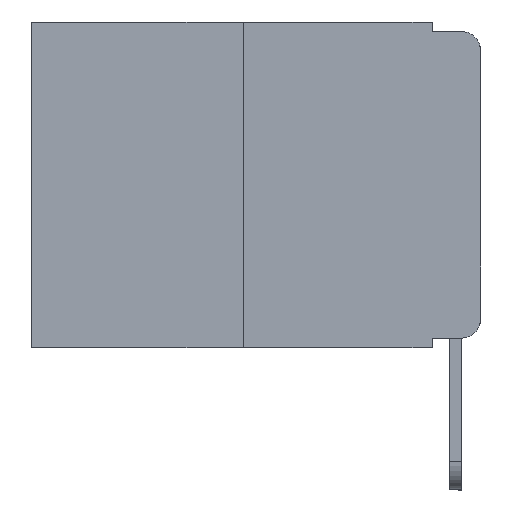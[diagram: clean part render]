
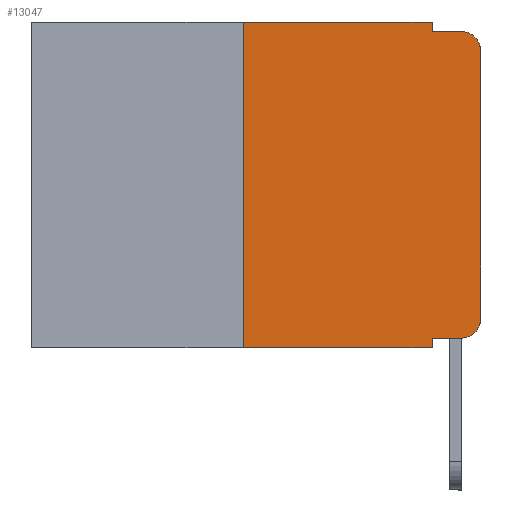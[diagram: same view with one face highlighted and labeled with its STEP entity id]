
A CAD part, left-side view. The second image highlights one B-rep face of the part: STEP entity #13047.
In plain terms, the highlighted planar face has unit normal (-1, 0, 0).
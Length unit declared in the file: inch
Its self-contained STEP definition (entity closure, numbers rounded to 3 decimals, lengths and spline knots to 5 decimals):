
#60 = CARTESIAN_POINT ( 'NONE',  ( 0., 0.02, -0.01 ) ) ;
#327 = FACE_OUTER_BOUND ( 'NONE', #13938, .T. ) ;
#675 = CARTESIAN_POINT ( 'NONE',  ( 0., 0., -0.313 ) ) ;
#951 = EDGE_CURVE ( 'NONE', #6253, #8660, #1093, .T. ) ;
#1003 = CARTESIAN_POINT ( 'NONE',  ( 0., 0., 0. ) ) ;
#1093 = LINE ( 'NONE', #10043, #1370 ) ;
#1110 = CARTESIAN_POINT ( 'NONE',  ( 0., 0.051, -0.333 ) ) ;
#1283 = DIRECTION ( 'NONE',  ( 0., 0., -1. ) ) ;
#1335 = CARTESIAN_POINT ( 'NONE',  ( 0., 0.051, -0.01 ) ) ;
#1370 = VECTOR ( 'NONE', #1283, 39.37008 ) ;
#1663 = ORIENTED_EDGE ( 'NONE', *, *, #7862, .T. ) ;
#1770 = VERTEX_POINT ( 'NONE', #11690 ) ;
#1880 = CIRCLE ( 'NONE', #13882, 0.02 ) ;
#1901 = VECTOR ( 'NONE', #13381, 39.37008 ) ;
#1945 = DIRECTION ( 'NONE',  ( 0., 0., -1. ) ) ;
#2068 = DIRECTION ( 'NONE',  ( -1., 0., 0. ) ) ;
#2071 = CARTESIAN_POINT ( 'NONE',  ( 0., 0.473, 0. ) ) ;
#2600 = EDGE_CURVE ( 'NONE', #15318, #6253, #12463, .T. ) ;
#2618 = DIRECTION ( 'NONE',  ( 0., 0., 1. ) ) ;
#3320 = DIRECTION ( 'NONE',  ( 0., 0., -1. ) ) ;
#3401 = LINE ( 'NONE', #13617, #16373 ) ;
#3673 = DIRECTION ( 'NONE',  ( 1., 0., 0. ) ) ;
#3693 = DIRECTION ( 'NONE',  ( 0., -1., 0. ) ) ;
#3809 = VECTOR ( 'NONE', #3693, 39.37008 ) ;
#4186 = AXIS2_PLACEMENT_3D ( 'NONE', #15248, #3673, #3320 ) ;
#4267 = CARTESIAN_POINT ( 'NONE',  ( 0., 0.02, -0.333 ) ) ;
#4283 = VECTOR ( 'NONE', #12015, 39.37008 ) ;
#4466 = EDGE_CURVE ( 'NONE', #13913, #15318, #17165, .T. ) ;
#4729 = CIRCLE ( 'NONE', #17966, 0.02 ) ;
#4837 = VERTEX_POINT ( 'NONE', #675 ) ;
#4962 = ORIENTED_EDGE ( 'NONE', *, *, #4466, .F. ) ;
#5260 = DIRECTION ( 'NONE',  ( 0., 0., -1. ) ) ;
#6099 = ORIENTED_EDGE ( 'NONE', *, *, #7632, .T. ) ;
#6197 = VERTEX_POINT ( 'NONE', #18984 ) ;
#6253 = VERTEX_POINT ( 'NONE', #16194 ) ;
#6338 = CARTESIAN_POINT ( 'NONE',  ( 0., 0.051, -0.333 ) ) ;
#6472 = EDGE_CURVE ( 'NONE', #10472, #4837, #4729, .T. ) ;
#6666 = ORIENTED_EDGE ( 'NONE', *, *, #14820, .F. ) ;
#6845 = CARTESIAN_POINT ( 'NONE',  ( 0., 0.25, 0. ) ) ;
#6918 = EDGE_CURVE ( 'NONE', #4837, #6197, #14202, .T. ) ;
#6941 = VECTOR ( 'NONE', #2618, 39.37008 ) ;
#7389 = CARTESIAN_POINT ( 'NONE',  ( 0., 0.25, 0. ) ) ;
#7553 = ORIENTED_EDGE ( 'NONE', *, *, #14374, .T. ) ;
#7632 = EDGE_CURVE ( 'NONE', #17494, #10472, #7686, .T. ) ;
#7686 = LINE ( 'NONE', #6338, #10735 ) ;
#7763 = ORIENTED_EDGE ( 'NONE', *, *, #951, .F. ) ;
#7862 = EDGE_CURVE ( 'NONE', #13913, #1770, #11926, .T. ) ;
#7932 = DIRECTION ( 'NONE',  ( 0., 0., -1. ) ) ;
#8291 = CARTESIAN_POINT ( 'NONE',  ( 0., 0.051, -0.01 ) ) ;
#8660 = VERTEX_POINT ( 'NONE', #8291 ) ;
#8730 = CARTESIAN_POINT ( 'NONE',  ( 0., 0.473, -0.343 ) ) ;
#9581 = VERTEX_POINT ( 'NONE', #60 ) ;
#9664 = DIRECTION ( 'NONE',  ( 0., 0., 1. ) ) ;
#9686 = DIRECTION ( 'NONE',  ( -1., 0., 0. ) ) ;
#10043 = CARTESIAN_POINT ( 'NONE',  ( 0., 0.051, 0. ) ) ;
#10136 = VECTOR ( 'NONE', #9664, 39.37008 ) ;
#10472 = VERTEX_POINT ( 'NONE', #4267 ) ;
#10631 = PLANE ( 'NONE',  #4186 ) ;
#10735 = VECTOR ( 'NONE', #12220, 39.37008 ) ;
#11314 = ORIENTED_EDGE ( 'NONE', *, *, #6918, .T. ) ;
#11690 = CARTESIAN_POINT ( 'NONE',  ( 0., 0.051, -0.343 ) ) ;
#11926 = LINE ( 'NONE', #8730, #4283 ) ;
#12015 = DIRECTION ( 'NONE',  ( 0., -1., 0. ) ) ;
#12044 = CARTESIAN_POINT ( 'NONE',  ( 0., 0.25, -0.343 ) ) ;
#12220 = DIRECTION ( 'NONE',  ( 0., -1., 0. ) ) ;
#12463 = LINE ( 'NONE', #2071, #3809 ) ;
#13047 = ADVANCED_FACE ( 'NONE', ( #327 ), #10631, .F. ) ;
#13238 = ORIENTED_EDGE ( 'NONE', *, *, #15304, .F. ) ;
#13381 = DIRECTION ( 'NONE',  ( 0., -1., 0. ) ) ;
#13617 = CARTESIAN_POINT ( 'NONE',  ( 0., 0.051, 0. ) ) ;
#13882 = AXIS2_PLACEMENT_3D ( 'NONE', #16541, #2068, #7932 ) ;
#13913 = VERTEX_POINT ( 'NONE', #12044 ) ;
#13938 = EDGE_LOOP ( 'NONE', ( #11314, #7553, #13238, #7763, #16247, #4962, #1663, #6666, #6099, #15882 ) ) ;
#14202 = LINE ( 'NONE', #1003, #10136 ) ;
#14323 = CARTESIAN_POINT ( 'NONE',  ( 0., 0.02, -0.313 ) ) ;
#14374 = EDGE_CURVE ( 'NONE', #6197, #9581, #1880, .T. ) ;
#14433 = LINE ( 'NONE', #1335, #1901 ) ;
#14820 = EDGE_CURVE ( 'NONE', #17494, #1770, #3401, .T. ) ;
#15248 = CARTESIAN_POINT ( 'NONE',  ( 0., 0.473, 0. ) ) ;
#15304 = EDGE_CURVE ( 'NONE', #8660, #9581, #14433, .T. ) ;
#15318 = VERTEX_POINT ( 'NONE', #7389 ) ;
#15882 = ORIENTED_EDGE ( 'NONE', *, *, #6472, .T. ) ;
#16194 = CARTESIAN_POINT ( 'NONE',  ( 0., 0.051, 0. ) ) ;
#16247 = ORIENTED_EDGE ( 'NONE', *, *, #2600, .F. ) ;
#16373 = VECTOR ( 'NONE', #1945, 39.37008 ) ;
#16541 = CARTESIAN_POINT ( 'NONE',  ( 0., 0.02, -0.03 ) ) ;
#17165 = LINE ( 'NONE', #6845, #6941 ) ;
#17494 = VERTEX_POINT ( 'NONE', #1110 ) ;
#17966 = AXIS2_PLACEMENT_3D ( 'NONE', #14323, #9686, #5260 ) ;
#18984 = CARTESIAN_POINT ( 'NONE',  ( 0., 0., -0.03 ) ) ;
